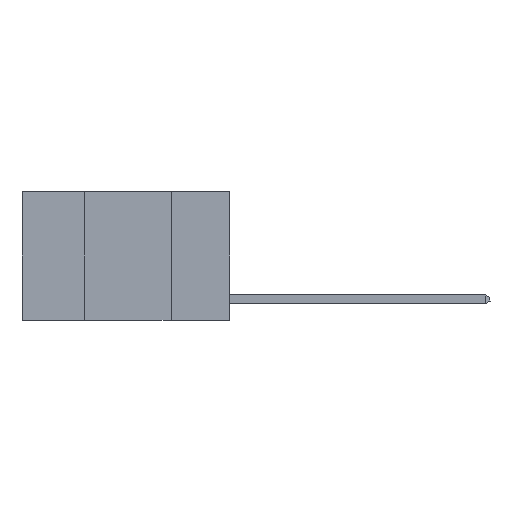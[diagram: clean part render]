
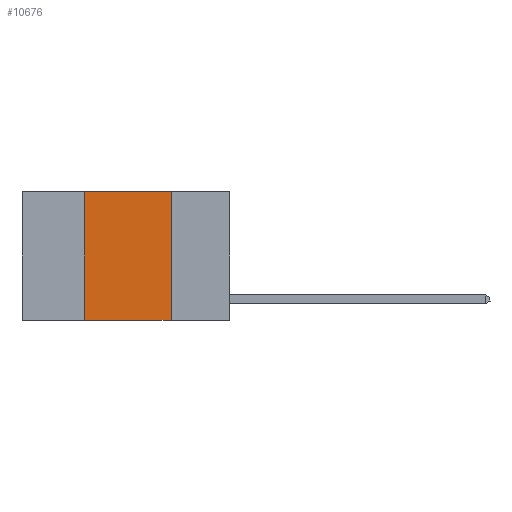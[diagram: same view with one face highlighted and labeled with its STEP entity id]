
A CAD part, left-side view. The second image highlights one B-rep face of the part: STEP entity #10676.
In plain terms, the highlighted planar face has unit normal (-1, 0, 0).
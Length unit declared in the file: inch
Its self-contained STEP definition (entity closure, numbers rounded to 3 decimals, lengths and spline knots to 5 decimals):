
#377 = LINE ( 'NONE', #661, #22575 ) ;
#485 = CARTESIAN_POINT ( 'NONE',  ( 0., 0.6, 0. ) ) ;
#661 = CARTESIAN_POINT ( 'NONE',  ( 0., 0.6, -0.37 ) ) ;
#1046 = VERTEX_POINT ( 'NONE', #6173 ) ;
#2014 = CARTESIAN_POINT ( 'NONE',  ( 0., 0.6, 0. ) ) ;
#2067 = EDGE_LOOP ( 'NONE', ( #13569, #2759, #17660, #11100 ) ) ;
#2759 = ORIENTED_EDGE ( 'NONE', *, *, #16923, .F. ) ;
#3434 = LINE ( 'NONE', #7619, #13562 ) ;
#4682 = DIRECTION ( 'NONE',  ( 1., 0., 0. ) ) ;
#5589 = VECTOR ( 'NONE', #19974, 39.37008 ) ;
#6173 = CARTESIAN_POINT ( 'NONE',  ( 0., 0.42, -0.37 ) ) ;
#7619 = CARTESIAN_POINT ( 'NONE',  ( 0., 0.17, 0. ) ) ;
#7755 = VECTOR ( 'NONE', #18225, 39.37008 ) ;
#7791 = CARTESIAN_POINT ( 'NONE',  ( 0., 0.42, 0. ) ) ;
#8831 = EDGE_CURVE ( 'NONE', #1046, #18664, #377, .T. ) ;
#9715 = EDGE_CURVE ( 'NONE', #1046, #18039, #11003, .T. ) ;
#10676 = ADVANCED_FACE ( 'NONE', ( #20338 ), #10757, .F. ) ;
#10757 = PLANE ( 'NONE',  #20377 ) ;
#11003 = LINE ( 'NONE', #7791, #5589 ) ;
#11100 = ORIENTED_EDGE ( 'NONE', *, *, #8831, .T. ) ;
#12904 = DIRECTION ( 'NONE',  ( 0., -1., 0. ) ) ;
#12976 = CARTESIAN_POINT ( 'NONE',  ( 0., 0.17, 0. ) ) ;
#13562 = VECTOR ( 'NONE', #21625, 39.37008 ) ;
#13569 = ORIENTED_EDGE ( 'NONE', *, *, #19552, .F. ) ;
#14685 = VERTEX_POINT ( 'NONE', #12976 ) ;
#15122 = CARTESIAN_POINT ( 'NONE',  ( 0., 0.42, 0. ) ) ;
#16923 = EDGE_CURVE ( 'NONE', #18039, #14685, #19670, .T. ) ;
#17660 = ORIENTED_EDGE ( 'NONE', *, *, #9715, .F. ) ;
#18039 = VERTEX_POINT ( 'NONE', #15122 ) ;
#18225 = DIRECTION ( 'NONE',  ( 0., -1., 0. ) ) ;
#18664 = VERTEX_POINT ( 'NONE', #22906 ) ;
#18766 = DIRECTION ( 'NONE',  ( 0., 0., -1. ) ) ;
#19552 = EDGE_CURVE ( 'NONE', #14685, #18664, #3434, .T. ) ;
#19670 = LINE ( 'NONE', #2014, #7755 ) ;
#19974 = DIRECTION ( 'NONE',  ( 0., 0., 1. ) ) ;
#20338 = FACE_OUTER_BOUND ( 'NONE', #2067, .T. ) ;
#20377 = AXIS2_PLACEMENT_3D ( 'NONE', #485, #4682, #18766 ) ;
#21625 = DIRECTION ( 'NONE',  ( 0., 0., -1. ) ) ;
#22575 = VECTOR ( 'NONE', #12904, 39.37008 ) ;
#22906 = CARTESIAN_POINT ( 'NONE',  ( 0., 0.17, -0.37 ) ) ;
